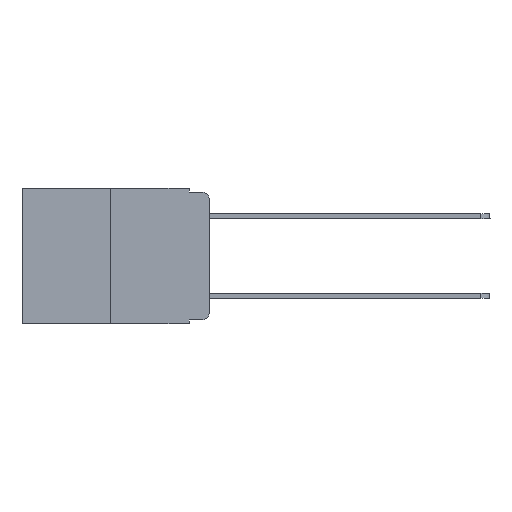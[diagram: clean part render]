
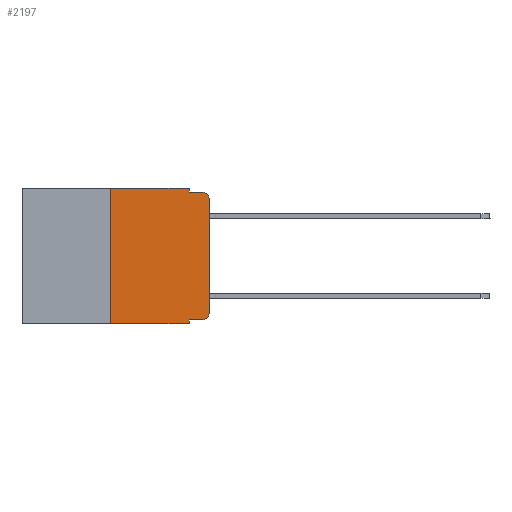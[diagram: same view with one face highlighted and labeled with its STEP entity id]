
A CAD part, left-side view. The second image highlights one B-rep face of the part: STEP entity #2197.
In plain terms, the highlighted planar face has unit normal (-1, 0, 0).
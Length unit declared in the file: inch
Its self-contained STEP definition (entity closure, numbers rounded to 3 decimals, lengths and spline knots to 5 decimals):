
#10 = VECTOR ( 'NONE', #22431, 39.37008 ) ;
#347 = VECTOR ( 'NONE', #18631, 39.37008 ) ;
#839 = LINE ( 'NONE', #19657, #21130 ) ;
#1174 = VERTEX_POINT ( 'NONE', #24584 ) ;
#1211 = EDGE_CURVE ( 'NONE', #24935, #15215, #10819, .T. ) ;
#1233 = DIRECTION ( 'NONE',  ( 0., 0., -1. ) ) ;
#2197 = ADVANCED_FACE ( 'NONE', ( #4112 ), #6152, .F. ) ;
#2216 = LINE ( 'NONE', #12425, #8263 ) ;
#2260 = EDGE_CURVE ( 'NONE', #15215, #20379, #19616, .T. ) ;
#2737 = CARTESIAN_POINT ( 'NONE',  ( 0., 0.051, -0.333 ) ) ;
#3118 = CARTESIAN_POINT ( 'NONE',  ( 0., 0., 0. ) ) ;
#3318 = VERTEX_POINT ( 'NONE', #21902 ) ;
#3974 = ORIENTED_EDGE ( 'NONE', *, *, #14143, .T. ) ;
#4112 = FACE_OUTER_BOUND ( 'NONE', #16516, .T. ) ;
#4497 = CARTESIAN_POINT ( 'NONE',  ( 0., 0.051, 0. ) ) ;
#4508 = VERTEX_POINT ( 'NONE', #18441 ) ;
#5284 = ORIENTED_EDGE ( 'NONE', *, *, #2260, .F. ) ;
#5332 = VERTEX_POINT ( 'NONE', #15039 ) ;
#5601 = AXIS2_PLACEMENT_3D ( 'NONE', #12238, #10133, #20289 ) ;
#5820 = EDGE_CURVE ( 'NONE', #15901, #3318, #12189, .T. ) ;
#6152 = PLANE ( 'NONE',  #5601 ) ;
#6332 = DIRECTION ( 'NONE',  ( 0., -1., 0. ) ) ;
#6848 = AXIS2_PLACEMENT_3D ( 'NONE', #23378, #25415, #1233 ) ;
#7156 = DIRECTION ( 'NONE',  ( 0., 0., -1. ) ) ;
#7209 = DIRECTION ( 'NONE',  ( 0., 0., 1. ) ) ;
#8263 = VECTOR ( 'NONE', #20814, 39.37008 ) ;
#8337 = VERTEX_POINT ( 'NONE', #2737 ) ;
#8880 = LINE ( 'NONE', #19254, #9827 ) ;
#9827 = VECTOR ( 'NONE', #7156, 39.37008 ) ;
#9944 = EDGE_CURVE ( 'NONE', #21062, #5332, #2216, .T. ) ;
#10133 = DIRECTION ( 'NONE',  ( 1., 0., 0. ) ) ;
#10616 = ORIENTED_EDGE ( 'NONE', *, *, #9944, .F. ) ;
#10819 = LINE ( 'NONE', #4497, #347 ) ;
#10834 = EDGE_CURVE ( 'NONE', #8337, #4508, #22481, .T. ) ;
#11114 = CARTESIAN_POINT ( 'NONE',  ( 0., 0.051, -0.01 ) ) ;
#11118 = ORIENTED_EDGE ( 'NONE', *, *, #16192, .F. ) ;
#12186 = EDGE_CURVE ( 'NONE', #21062, #1174, #839, .T. ) ;
#12189 = LINE ( 'NONE', #3118, #22005 ) ;
#12238 = CARTESIAN_POINT ( 'NONE',  ( 0., 0.473, 0. ) ) ;
#12425 = CARTESIAN_POINT ( 'NONE',  ( 0., 0.25, 0. ) ) ;
#13613 = VECTOR ( 'NONE', #26001, 39.37008 ) ;
#13766 = CARTESIAN_POINT ( 'NONE',  ( 0., 0., -0.313 ) ) ;
#14143 = EDGE_CURVE ( 'NONE', #3318, #20379, #15032, .T. ) ;
#14187 = CARTESIAN_POINT ( 'NONE',  ( 0., 0.25, -0.343 ) ) ;
#14456 = CARTESIAN_POINT ( 'NONE',  ( 0., 0.473, 0. ) ) ;
#15032 = CIRCLE ( 'NONE', #6848, 0.02 ) ;
#15039 = CARTESIAN_POINT ( 'NONE',  ( 0., 0.25, 0. ) ) ;
#15215 = VERTEX_POINT ( 'NONE', #11114 ) ;
#15440 = ORIENTED_EDGE ( 'NONE', *, *, #1211, .F. ) ;
#15684 = DIRECTION ( 'NONE',  ( -1., 0., 0. ) ) ;
#15901 = VERTEX_POINT ( 'NONE', #13766 ) ;
#16050 = CARTESIAN_POINT ( 'NONE',  ( 0., 0.051, -0.333 ) ) ;
#16192 = EDGE_CURVE ( 'NONE', #5332, #24935, #26018, .T. ) ;
#16516 = EDGE_LOOP ( 'NONE', ( #24955, #3974, #5284, #15440, #11118, #10616, #22044, #22558, #19564, #25714 ) ) ;
#17527 = EDGE_CURVE ( 'NONE', #8337, #1174, #8880, .T. ) ;
#17786 = DIRECTION ( 'NONE',  ( 0., -1., 0. ) ) ;
#18441 = CARTESIAN_POINT ( 'NONE',  ( 0., 0.02, -0.333 ) ) ;
#18631 = DIRECTION ( 'NONE',  ( 0., 0., -1. ) ) ;
#19006 = EDGE_CURVE ( 'NONE', #4508, #15901, #19553, .T. ) ;
#19254 = CARTESIAN_POINT ( 'NONE',  ( 0., 0.051, 0. ) ) ;
#19422 = CARTESIAN_POINT ( 'NONE',  ( 0., 0.02, -0.313 ) ) ;
#19553 = CIRCLE ( 'NONE', #22672, 0.02 ) ;
#19564 = ORIENTED_EDGE ( 'NONE', *, *, #10834, .T. ) ;
#19616 = LINE ( 'NONE', #22417, #24381 ) ;
#19657 = CARTESIAN_POINT ( 'NONE',  ( 0., 0.473, -0.343 ) ) ;
#19659 = CARTESIAN_POINT ( 'NONE',  ( 0., 0.051, 0. ) ) ;
#20289 = DIRECTION ( 'NONE',  ( 0., 0., -1. ) ) ;
#20379 = VERTEX_POINT ( 'NONE', #22291 ) ;
#20814 = DIRECTION ( 'NONE',  ( 0., 0., 1. ) ) ;
#21062 = VERTEX_POINT ( 'NONE', #14187 ) ;
#21130 = VECTOR ( 'NONE', #17786, 39.37008 ) ;
#21554 = DIRECTION ( 'NONE',  ( 0., 0., -1. ) ) ;
#21902 = CARTESIAN_POINT ( 'NONE',  ( 0., 0., -0.03 ) ) ;
#22005 = VECTOR ( 'NONE', #7209, 39.37008 ) ;
#22044 = ORIENTED_EDGE ( 'NONE', *, *, #12186, .T. ) ;
#22291 = CARTESIAN_POINT ( 'NONE',  ( 0., 0.02, -0.01 ) ) ;
#22417 = CARTESIAN_POINT ( 'NONE',  ( 0., 0.051, -0.01 ) ) ;
#22431 = DIRECTION ( 'NONE',  ( 0., -1., 0. ) ) ;
#22481 = LINE ( 'NONE', #16050, #13613 ) ;
#22558 = ORIENTED_EDGE ( 'NONE', *, *, #17527, .F. ) ;
#22672 = AXIS2_PLACEMENT_3D ( 'NONE', #19422, #15684, #21554 ) ;
#23378 = CARTESIAN_POINT ( 'NONE',  ( 0., 0.02, -0.03 ) ) ;
#24381 = VECTOR ( 'NONE', #6332, 39.37008 ) ;
#24584 = CARTESIAN_POINT ( 'NONE',  ( 0., 0.051, -0.343 ) ) ;
#24935 = VERTEX_POINT ( 'NONE', #19659 ) ;
#24955 = ORIENTED_EDGE ( 'NONE', *, *, #5820, .T. ) ;
#25415 = DIRECTION ( 'NONE',  ( -1., 0., 0. ) ) ;
#25714 = ORIENTED_EDGE ( 'NONE', *, *, #19006, .T. ) ;
#26001 = DIRECTION ( 'NONE',  ( 0., -1., 0. ) ) ;
#26018 = LINE ( 'NONE', #14456, #10 ) ;
